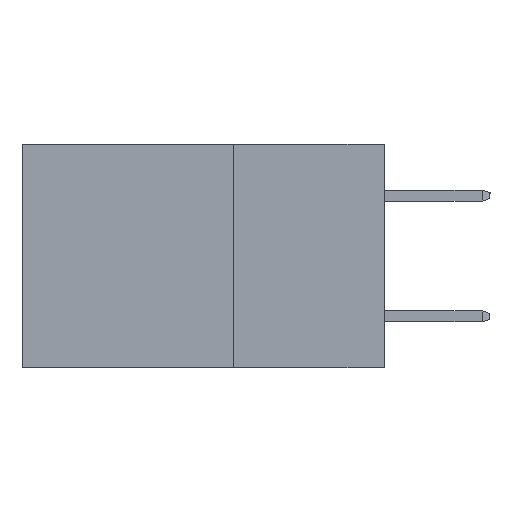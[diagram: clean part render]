
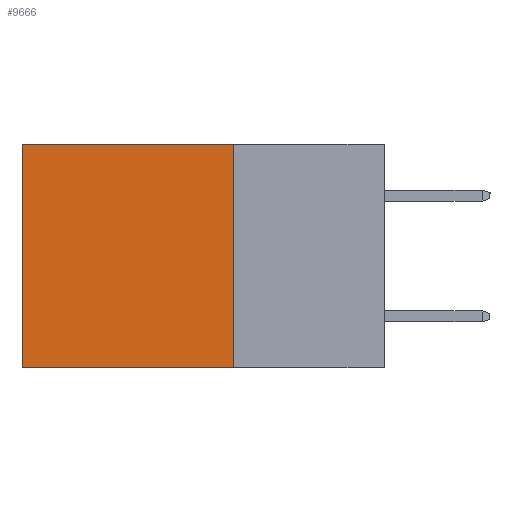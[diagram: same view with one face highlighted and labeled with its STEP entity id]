
A CAD part, left-side view. The second image highlights one B-rep face of the part: STEP entity #9666.
In plain terms, the highlighted planar face has unit normal (-1, 0, 0).
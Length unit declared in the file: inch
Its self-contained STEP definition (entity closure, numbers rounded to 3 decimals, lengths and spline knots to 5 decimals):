
#1003 = CARTESIAN_POINT ( 'NONE',  ( 0.2615, 0.25, 0. ) ) ;
#1873 = LINE ( 'NONE', #19013, #24370 ) ;
#2099 = VECTOR ( 'NONE', #11723, 39.37008 ) ;
#2189 = EDGE_CURVE ( 'NONE', #6836, #11618, #23671, .T. ) ;
#2730 = FACE_OUTER_BOUND ( 'NONE', #9665, .T. ) ;
#3074 = LINE ( 'NONE', #10638, #15409 ) ;
#4155 = LINE ( 'NONE', #9604, #2099 ) ;
#4536 = EDGE_CURVE ( 'NONE', #11024, #6836, #3074, .T. ) ;
#4727 = ORIENTED_EDGE ( 'NONE', *, *, #16320, .T. ) ;
#6836 = VERTEX_POINT ( 'NONE', #19323 ) ;
#9125 = CARTESIAN_POINT ( 'NONE',  ( 0.2615, 0.6, -0.37 ) ) ;
#9158 = ORIENTED_EDGE ( 'NONE', *, *, #4536, .F. ) ;
#9440 = DIRECTION ( 'NONE',  ( 0., 1., 0. ) ) ;
#9604 = CARTESIAN_POINT ( 'NONE',  ( 0.2615, 0.6, -0.37 ) ) ;
#9632 = ORIENTED_EDGE ( 'NONE', *, *, #15418, .T. ) ;
#9665 = EDGE_LOOP ( 'NONE', ( #9632, #15996, #9158, #4727 ) ) ;
#9666 = ADVANCED_FACE ( 'NONE', ( #2730 ), #10658, .F. ) ;
#9748 = AXIS2_PLACEMENT_3D ( 'NONE', #17865, #18117, #18239 ) ;
#10638 = CARTESIAN_POINT ( 'NONE',  ( 0.2615, 0.25, -0.37 ) ) ;
#10658 = PLANE ( 'NONE',  #9748 ) ;
#11024 = VERTEX_POINT ( 'NONE', #1003 ) ;
#11618 = VERTEX_POINT ( 'NONE', #9125 ) ;
#11723 = DIRECTION ( 'NONE',  ( 0., 0., -1. ) ) ;
#12221 = DIRECTION ( 'NONE',  ( 0., 1., 0. ) ) ;
#14418 = VECTOR ( 'NONE', #12221, 39.37008 ) ;
#15409 = VECTOR ( 'NONE', #24296, 39.37008 ) ;
#15418 = EDGE_CURVE ( 'NONE', #24289, #11618, #4155, .T. ) ;
#15647 = CARTESIAN_POINT ( 'NONE',  ( 0.2615, 0.6, 0. ) ) ;
#15695 = CARTESIAN_POINT ( 'NONE',  ( 0.2615, 0.25, -0.37 ) ) ;
#15996 = ORIENTED_EDGE ( 'NONE', *, *, #2189, .F. ) ;
#16320 = EDGE_CURVE ( 'NONE', #11024, #24289, #1873, .T. ) ;
#17865 = CARTESIAN_POINT ( 'NONE',  ( 0.2615, 0.25, -0.37 ) ) ;
#18117 = DIRECTION ( 'NONE',  ( 1., 0., 0. ) ) ;
#18239 = DIRECTION ( 'NONE',  ( 0., 0., -1. ) ) ;
#19013 = CARTESIAN_POINT ( 'NONE',  ( 0.2615, 0.25, 0. ) ) ;
#19323 = CARTESIAN_POINT ( 'NONE',  ( 0.2615, 0.25, -0.37 ) ) ;
#23671 = LINE ( 'NONE', #15695, #14418 ) ;
#24289 = VERTEX_POINT ( 'NONE', #15647 ) ;
#24296 = DIRECTION ( 'NONE',  ( 0., 0., -1. ) ) ;
#24370 = VECTOR ( 'NONE', #9440, 39.37008 ) ;
